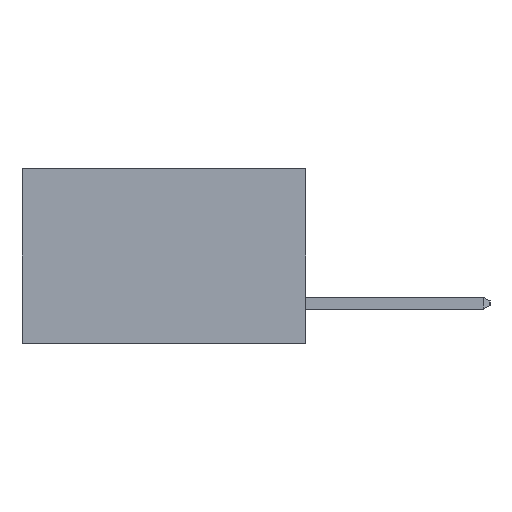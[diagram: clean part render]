
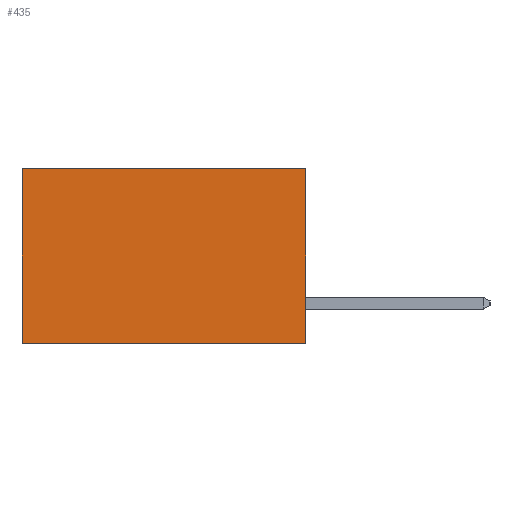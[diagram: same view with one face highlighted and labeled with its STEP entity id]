
A CAD part, left-side view. The second image highlights one B-rep face of the part: STEP entity #435.
In plain terms, the highlighted planar face has unit normal (-1, 0, 0).
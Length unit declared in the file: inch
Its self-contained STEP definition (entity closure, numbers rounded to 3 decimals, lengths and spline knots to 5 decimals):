
#435 = ADVANCED_FACE ( 'NONE', ( #2911 ), #8901, .F. ) ;
#1235 = DIRECTION ( 'NONE',  ( 0., 0., -1. ) ) ;
#1318 = CARTESIAN_POINT ( 'NONE',  ( 0.298, 0., 0. ) ) ;
#1836 = CARTESIAN_POINT ( 'NONE',  ( 0.298, 0., 0. ) ) ;
#2038 = DIRECTION ( 'NONE',  ( 0., 1., 0. ) ) ;
#2416 = VECTOR ( 'NONE', #2038, 39.37008 ) ;
#2482 = CARTESIAN_POINT ( 'NONE',  ( 0.298, 0.6, -0.37 ) ) ;
#2542 = LINE ( 'NONE', #12177, #13395 ) ;
#2911 = FACE_OUTER_BOUND ( 'NONE', #13306, .T. ) ;
#2946 = CARTESIAN_POINT ( 'NONE',  ( 0.298, 0.6, 0. ) ) ;
#3062 = EDGE_CURVE ( 'NONE', #6810, #5158, #8065, .T. ) ;
#3172 = ORIENTED_EDGE ( 'NONE', *, *, #4998, .F. ) ;
#4028 = DIRECTION ( 'NONE',  ( 0., 0., -1. ) ) ;
#4126 = EDGE_CURVE ( 'NONE', #6810, #6005, #2542, .T. ) ;
#4998 = EDGE_CURVE ( 'NONE', #6005, #8667, #11007, .T. ) ;
#5158 = VERTEX_POINT ( 'NONE', #12783 ) ;
#5697 = VECTOR ( 'NONE', #11893, 39.37008 ) ;
#5912 = ORIENTED_EDGE ( 'NONE', *, *, #4126, .F. ) ;
#6005 = VERTEX_POINT ( 'NONE', #12756 ) ;
#6748 = DIRECTION ( 'NONE',  ( 0., 0., -1. ) ) ;
#6780 = CARTESIAN_POINT ( 'NONE',  ( 0.298, 0., 0. ) ) ;
#6810 = VERTEX_POINT ( 'NONE', #6780 ) ;
#7255 = DIRECTION ( 'NONE',  ( 1., 0., 0. ) ) ;
#7314 = CARTESIAN_POINT ( 'NONE',  ( 0.298, 0., -0.37 ) ) ;
#8065 = LINE ( 'NONE', #1836, #2416 ) ;
#8246 = ORIENTED_EDGE ( 'NONE', *, *, #11685, .T. ) ;
#8303 = ORIENTED_EDGE ( 'NONE', *, *, #3062, .T. ) ;
#8667 = VERTEX_POINT ( 'NONE', #2482 ) ;
#8901 = PLANE ( 'NONE',  #9538 ) ;
#9538 = AXIS2_PLACEMENT_3D ( 'NONE', #1318, #7255, #1235 ) ;
#11007 = LINE ( 'NONE', #7314, #5697 ) ;
#11685 = EDGE_CURVE ( 'NONE', #5158, #8667, #12645, .T. ) ;
#11893 = DIRECTION ( 'NONE',  ( 0., 1., 0. ) ) ;
#12177 = CARTESIAN_POINT ( 'NONE',  ( 0.298, 0., 0. ) ) ;
#12335 = VECTOR ( 'NONE', #4028, 39.37008 ) ;
#12645 = LINE ( 'NONE', #2946, #12335 ) ;
#12756 = CARTESIAN_POINT ( 'NONE',  ( 0.298, 0., -0.37 ) ) ;
#12783 = CARTESIAN_POINT ( 'NONE',  ( 0.298, 0.6, 0. ) ) ;
#13306 = EDGE_LOOP ( 'NONE', ( #8246, #3172, #5912, #8303 ) ) ;
#13395 = VECTOR ( 'NONE', #6748, 39.37008 ) ;
